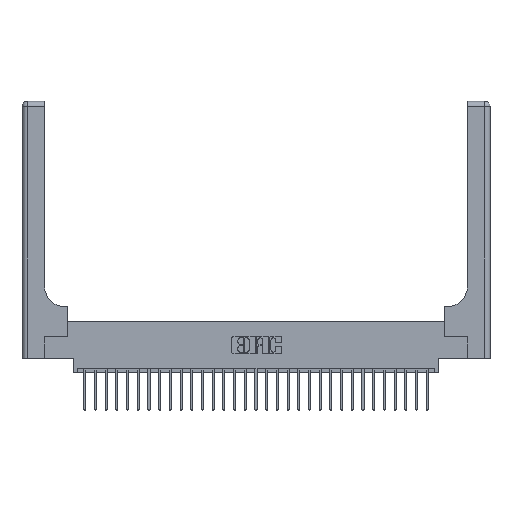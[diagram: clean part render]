
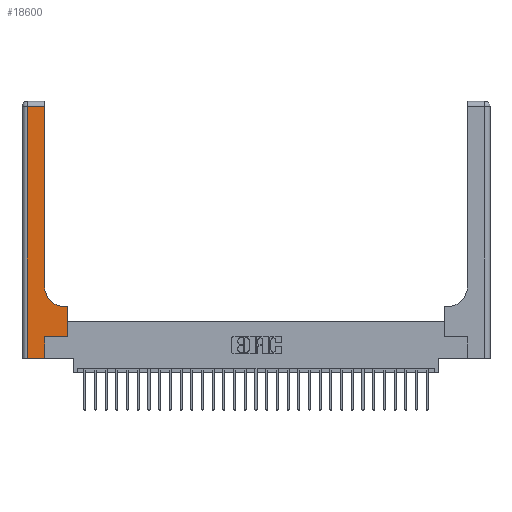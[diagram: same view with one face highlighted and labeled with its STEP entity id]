
A CAD part, top view. The second image highlights one B-rep face of the part: STEP entity #18600.
In plain terms, the highlighted planar face has unit normal (0, 0, 1).
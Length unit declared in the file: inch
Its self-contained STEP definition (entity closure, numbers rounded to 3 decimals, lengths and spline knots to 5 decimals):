
#142 = CARTESIAN_POINT ( 'NONE',  ( 0.51, 0.6, 0.37 ) ) ;
#514 = CIRCLE ( 'NONE', #5604, 0.25 ) ;
#1164 = VECTOR ( 'NONE', #20490, 39.37008 ) ;
#1202 = LINE ( 'NONE', #14465, #1349 ) ;
#1349 = VECTOR ( 'NONE', #27615, 39.37008 ) ;
#1392 = EDGE_CURVE ( 'NONE', #17060, #2774, #514, .T. ) ;
#1421 = DIRECTION ( 'NONE',  ( 0., -1., 0. ) ) ;
#1909 = EDGE_CURVE ( 'NONE', #19577, #3365, #23631, .T. ) ;
#2576 = VECTOR ( 'NONE', #23131, 39.37008 ) ;
#2774 = VERTEX_POINT ( 'NONE', #19108 ) ;
#2890 = CARTESIAN_POINT ( 'NONE',  ( 0.265, 0., 0.37 ) ) ;
#3365 = VERTEX_POINT ( 'NONE', #21091 ) ;
#3479 = FACE_OUTER_BOUND ( 'NONE', #8721, .T. ) ;
#4816 = LINE ( 'NONE', #20553, #9374 ) ;
#4818 = DIRECTION ( 'NONE',  ( 0., 0., -1. ) ) ;
#5087 = VERTEX_POINT ( 'NONE', #9450 ) ;
#5490 = CARTESIAN_POINT ( 'NONE',  ( 0.26, 2.94, 0.37 ) ) ;
#5604 = AXIS2_PLACEMENT_3D ( 'NONE', #9582, #4818, #18086 ) ;
#5630 = DIRECTION ( 'NONE',  ( 0., 0., -1. ) ) ;
#5749 = DIRECTION ( 'NONE',  ( 1., 0., 0. ) ) ;
#5885 = LINE ( 'NONE', #25798, #6973 ) ;
#6079 = CARTESIAN_POINT ( 'NONE',  ( 0.265, 0.25, 0.37 ) ) ;
#6659 = EDGE_CURVE ( 'NONE', #19328, #14472, #5885, .T. ) ;
#6924 = DIRECTION ( 'NONE',  ( -1., 0., 0. ) ) ;
#6973 = VECTOR ( 'NONE', #1421, 39.37008 ) ;
#7668 = AXIS2_PLACEMENT_3D ( 'NONE', #25395, #5630, #12261 ) ;
#7937 = ORIENTED_EDGE ( 'NONE', *, *, #6659, .T. ) ;
#8115 = CARTESIAN_POINT ( 'NONE',  ( 0.528, 0.6, 0.37 ) ) ;
#8191 = ORIENTED_EDGE ( 'NONE', *, *, #14968, .T. ) ;
#8721 = EDGE_LOOP ( 'NONE', ( #13448, #23508, #7937, #15112, #8191, #10279, #28297, #21827, #24964 ) ) ;
#8976 = CARTESIAN_POINT ( 'NONE',  ( 0.06, 0., 0.37 ) ) ;
#9374 = VECTOR ( 'NONE', #13470, 39.37008 ) ;
#9450 = CARTESIAN_POINT ( 'NONE',  ( 0.265, 0., 0.37 ) ) ;
#9582 = CARTESIAN_POINT ( 'NONE',  ( 0.51, 0.85, 0.37 ) ) ;
#9605 = VERTEX_POINT ( 'NONE', #8115 ) ;
#9997 = VECTOR ( 'NONE', #19919, 39.37008 ) ;
#10279 = ORIENTED_EDGE ( 'NONE', *, *, #1909, .T. ) ;
#10512 = EDGE_CURVE ( 'NONE', #2774, #12068, #4816, .T. ) ;
#11262 = LINE ( 'NONE', #2890, #9997 ) ;
#12068 = VERTEX_POINT ( 'NONE', #5490 ) ;
#12261 = DIRECTION ( 'NONE',  ( -1., 0., 0. ) ) ;
#13448 = ORIENTED_EDGE ( 'NONE', *, *, #10512, .T. ) ;
#13470 = DIRECTION ( 'NONE',  ( 0., 1., 0. ) ) ;
#13971 = LINE ( 'NONE', #14277, #1164 ) ;
#14277 = CARTESIAN_POINT ( 'NONE',  ( 0., 0., 0.37 ) ) ;
#14465 = CARTESIAN_POINT ( 'NONE',  ( 0.26, 0.6, 0.37 ) ) ;
#14472 = VERTEX_POINT ( 'NONE', #8976 ) ;
#14968 = EDGE_CURVE ( 'NONE', #5087, #19577, #11262, .T. ) ;
#15112 = ORIENTED_EDGE ( 'NONE', *, *, #25009, .T. ) ;
#15777 = EDGE_CURVE ( 'NONE', #9605, #17060, #1202, .T. ) ;
#16066 = VECTOR ( 'NONE', #6924, 39.37008 ) ;
#16604 = PLANE ( 'NONE',  #7668 ) ;
#17060 = VERTEX_POINT ( 'NONE', #142 ) ;
#17293 = CARTESIAN_POINT ( 'NONE',  ( 0.265, 0.25, 0.37 ) ) ;
#18086 = DIRECTION ( 'NONE',  ( 1., 0., 0. ) ) ;
#18377 = CARTESIAN_POINT ( 'NONE',  ( 0.06, 2.94, 0.37 ) ) ;
#18600 = ADVANCED_FACE ( 'NONE', ( #3479 ), #16604, .F. ) ;
#19108 = CARTESIAN_POINT ( 'NONE',  ( 0.26, 0.85, 0.37 ) ) ;
#19328 = VERTEX_POINT ( 'NONE', #18377 ) ;
#19351 = EDGE_CURVE ( 'NONE', #3365, #9605, #25713, .T. ) ;
#19577 = VERTEX_POINT ( 'NONE', #6079 ) ;
#19730 = EDGE_CURVE ( 'NONE', #12068, #19328, #20358, .T. ) ;
#19919 = DIRECTION ( 'NONE',  ( 0., 1., 0. ) ) ;
#20358 = LINE ( 'NONE', #26699, #16066 ) ;
#20490 = DIRECTION ( 'NONE',  ( 1., 0., 0. ) ) ;
#20553 = CARTESIAN_POINT ( 'NONE',  ( 0.26, 3., 0.37 ) ) ;
#20912 = VECTOR ( 'NONE', #5749, 39.37008 ) ;
#21091 = CARTESIAN_POINT ( 'NONE',  ( 0.528, 0.25, 0.37 ) ) ;
#21827 = ORIENTED_EDGE ( 'NONE', *, *, #15777, .T. ) ;
#23131 = DIRECTION ( 'NONE',  ( 0., 1., 0. ) ) ;
#23508 = ORIENTED_EDGE ( 'NONE', *, *, #19730, .T. ) ;
#23631 = LINE ( 'NONE', #17293, #20912 ) ;
#24964 = ORIENTED_EDGE ( 'NONE', *, *, #1392, .T. ) ;
#25009 = EDGE_CURVE ( 'NONE', #14472, #5087, #13971, .T. ) ;
#25395 = CARTESIAN_POINT ( 'NONE',  ( 0., 3., 0.37 ) ) ;
#25434 = CARTESIAN_POINT ( 'NONE',  ( 0.528, 0.25, 0.37 ) ) ;
#25713 = LINE ( 'NONE', #25434, #2576 ) ;
#25798 = CARTESIAN_POINT ( 'NONE',  ( 0.06, 3., 0.37 ) ) ;
#26699 = CARTESIAN_POINT ( 'NONE',  ( 0., 2.94, 0.37 ) ) ;
#27615 = DIRECTION ( 'NONE',  ( -1., 0., 0. ) ) ;
#28297 = ORIENTED_EDGE ( 'NONE', *, *, #19351, .T. ) ;
